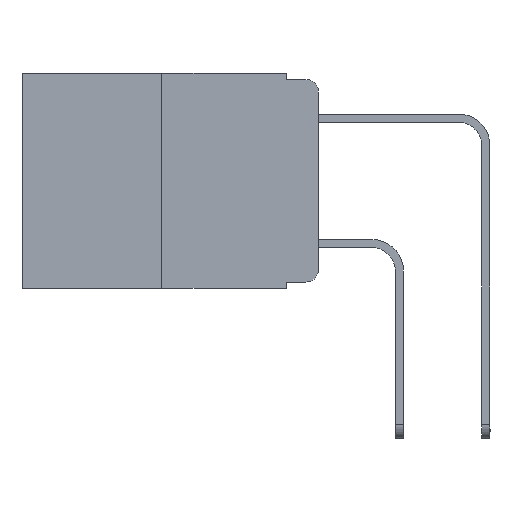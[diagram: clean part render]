
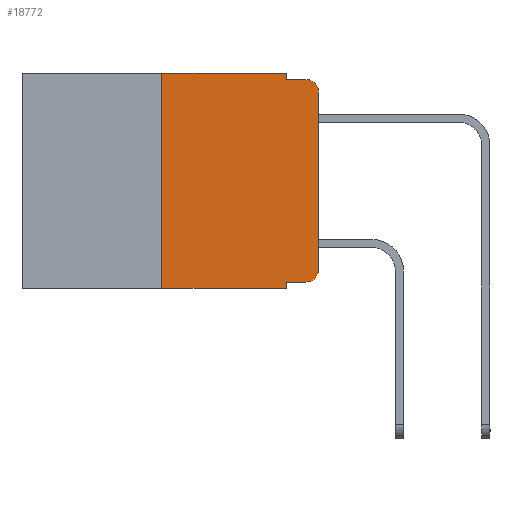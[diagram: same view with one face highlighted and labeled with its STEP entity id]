
A CAD part, left-side view. The second image highlights one B-rep face of the part: STEP entity #18772.
In plain terms, the highlighted planar face has unit normal (-1, 0, 0).
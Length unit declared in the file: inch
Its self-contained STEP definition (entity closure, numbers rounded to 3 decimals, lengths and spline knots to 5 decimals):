
#308 = DIRECTION ( 'NONE',  ( 0., 0., 1. ) ) ;
#322 = CARTESIAN_POINT ( 'NONE',  ( 0., 0.02, -0.333 ) ) ;
#410 = CARTESIAN_POINT ( 'NONE',  ( 0., 0.02, -0.313 ) ) ;
#515 = VECTOR ( 'NONE', #24752, 39.37008 ) ;
#552 = ORIENTED_EDGE ( 'NONE', *, *, #26550, .F. ) ;
#1046 = ORIENTED_EDGE ( 'NONE', *, *, #3903, .F. ) ;
#1959 = LINE ( 'NONE', #11991, #515 ) ;
#2117 = CARTESIAN_POINT ( 'NONE',  ( 0., 0.473, -0.343 ) ) ;
#2795 = VECTOR ( 'NONE', #3805, 39.37008 ) ;
#3055 = CARTESIAN_POINT ( 'NONE',  ( 0., 0.473, 0. ) ) ;
#3255 = CARTESIAN_POINT ( 'NONE',  ( 0., 0.051, -0.333 ) ) ;
#3805 = DIRECTION ( 'NONE',  ( 0., 0., -1. ) ) ;
#3903 = EDGE_CURVE ( 'NONE', #21490, #16347, #20404, .T. ) ;
#4224 = ORIENTED_EDGE ( 'NONE', *, *, #7014, .T. ) ;
#4335 = CARTESIAN_POINT ( 'NONE',  ( 0., 0., 0. ) ) ;
#4472 = LINE ( 'NONE', #4335, #6019 ) ;
#4534 = LINE ( 'NONE', #2117, #24745 ) ;
#4880 = AXIS2_PLACEMENT_3D ( 'NONE', #410, #16903, #4992 ) ;
#4992 = DIRECTION ( 'NONE',  ( 0., 0., -1. ) ) ;
#5060 = FACE_OUTER_BOUND ( 'NONE', #17353, .T. ) ;
#5159 = ORIENTED_EDGE ( 'NONE', *, *, #9480, .T. ) ;
#5389 = CARTESIAN_POINT ( 'NONE',  ( 0., 0.051, 0. ) ) ;
#5534 = DIRECTION ( 'NONE',  ( 0., 0., 1. ) ) ;
#6019 = VECTOR ( 'NONE', #308, 39.37008 ) ;
#6514 = ORIENTED_EDGE ( 'NONE', *, *, #7941, .F. ) ;
#7014 = EDGE_CURVE ( 'NONE', #9613, #23124, #14364, .T. ) ;
#7028 = VERTEX_POINT ( 'NONE', #19539 ) ;
#7389 = CARTESIAN_POINT ( 'NONE',  ( 0., 0.25, 0. ) ) ;
#7739 = ORIENTED_EDGE ( 'NONE', *, *, #18640, .T. ) ;
#7941 = EDGE_CURVE ( 'NONE', #16510, #10503, #19343, .T. ) ;
#8478 = VERTEX_POINT ( 'NONE', #9923 ) ;
#8979 = EDGE_CURVE ( 'NONE', #8478, #23124, #1959, .T. ) ;
#9098 = CARTESIAN_POINT ( 'NONE',  ( 0., 0.02, -0.01 ) ) ;
#9327 = DIRECTION ( 'NONE',  ( 1., 0., 0. ) ) ;
#9480 = EDGE_CURVE ( 'NONE', #16824, #7028, #12989, .T. ) ;
#9613 = VERTEX_POINT ( 'NONE', #15568 ) ;
#9795 = LINE ( 'NONE', #14210, #12015 ) ;
#9923 = CARTESIAN_POINT ( 'NONE',  ( 0., 0.051, -0.01 ) ) ;
#10267 = DIRECTION ( 'NONE',  ( 0., -1., 0. ) ) ;
#10503 = VERTEX_POINT ( 'NONE', #20475 ) ;
#11470 = PLANE ( 'NONE',  #24806 ) ;
#11743 = VECTOR ( 'NONE', #5534, 39.37008 ) ;
#11991 = CARTESIAN_POINT ( 'NONE',  ( 0., 0.051, -0.01 ) ) ;
#12015 = VECTOR ( 'NONE', #17972, 39.37008 ) ;
#12232 = CARTESIAN_POINT ( 'NONE',  ( 0., 0.051, 0. ) ) ;
#12686 = CARTESIAN_POINT ( 'NONE',  ( 0., 0.051, -0.343 ) ) ;
#12989 = CIRCLE ( 'NONE', #4880, 0.02 ) ;
#13209 = CARTESIAN_POINT ( 'NONE',  ( 0., 0.25, -0.343 ) ) ;
#13210 = ORIENTED_EDGE ( 'NONE', *, *, #8979, .F. ) ;
#14210 = CARTESIAN_POINT ( 'NONE',  ( 0., 0.051, 0. ) ) ;
#14364 = CIRCLE ( 'NONE', #23330, 0.02 ) ;
#15510 = DIRECTION ( 'NONE',  ( -1., 0., 0. ) ) ;
#15555 = DIRECTION ( 'NONE',  ( 0., -1., 0. ) ) ;
#15568 = CARTESIAN_POINT ( 'NONE',  ( 0., 0., -0.03 ) ) ;
#16347 = VERTEX_POINT ( 'NONE', #12686 ) ;
#16510 = VERTEX_POINT ( 'NONE', #13209 ) ;
#16783 = CARTESIAN_POINT ( 'NONE',  ( 0., 0.473, 0. ) ) ;
#16824 = VERTEX_POINT ( 'NONE', #322 ) ;
#16853 = ORIENTED_EDGE ( 'NONE', *, *, #21979, .T. ) ;
#16903 = DIRECTION ( 'NONE',  ( -1., 0., 0. ) ) ;
#16919 = LINE ( 'NONE', #16783, #18883 ) ;
#17353 = EDGE_LOOP ( 'NONE', ( #16853, #4224, #13210, #552, #26193, #6514, #7739, #1046, #21840, #5159 ) ) ;
#17803 = CARTESIAN_POINT ( 'NONE',  ( 0., 0.02, -0.03 ) ) ;
#17972 = DIRECTION ( 'NONE',  ( 0., 0., -1. ) ) ;
#18640 = EDGE_CURVE ( 'NONE', #16510, #16347, #4534, .T. ) ;
#18772 = ADVANCED_FACE ( 'NONE', ( #5060 ), #11470, .F. ) ;
#18883 = VECTOR ( 'NONE', #24995, 39.37008 ) ;
#19343 = LINE ( 'NONE', #7389, #11743 ) ;
#19385 = DIRECTION ( 'NONE',  ( 0., 0., -1. ) ) ;
#19539 = CARTESIAN_POINT ( 'NONE',  ( 0., 0., -0.313 ) ) ;
#20404 = LINE ( 'NONE', #12232, #2795 ) ;
#20475 = CARTESIAN_POINT ( 'NONE',  ( 0., 0.25, 0. ) ) ;
#21490 = VERTEX_POINT ( 'NONE', #26275 ) ;
#21819 = DIRECTION ( 'NONE',  ( 0., 0., -1. ) ) ;
#21840 = ORIENTED_EDGE ( 'NONE', *, *, #25826, .T. ) ;
#21979 = EDGE_CURVE ( 'NONE', #7028, #9613, #4472, .T. ) ;
#22005 = LINE ( 'NONE', #3255, #24438 ) ;
#23124 = VERTEX_POINT ( 'NONE', #9098 ) ;
#23330 = AXIS2_PLACEMENT_3D ( 'NONE', #17803, #15510, #21819 ) ;
#24438 = VECTOR ( 'NONE', #15555, 39.37008 ) ;
#24524 = VERTEX_POINT ( 'NONE', #5389 ) ;
#24745 = VECTOR ( 'NONE', #10267, 39.37008 ) ;
#24752 = DIRECTION ( 'NONE',  ( 0., -1., 0. ) ) ;
#24806 = AXIS2_PLACEMENT_3D ( 'NONE', #3055, #9327, #19385 ) ;
#24995 = DIRECTION ( 'NONE',  ( 0., -1., 0. ) ) ;
#25616 = EDGE_CURVE ( 'NONE', #10503, #24524, #16919, .T. ) ;
#25826 = EDGE_CURVE ( 'NONE', #21490, #16824, #22005, .T. ) ;
#26193 = ORIENTED_EDGE ( 'NONE', *, *, #25616, .F. ) ;
#26275 = CARTESIAN_POINT ( 'NONE',  ( 0., 0.051, -0.333 ) ) ;
#26550 = EDGE_CURVE ( 'NONE', #24524, #8478, #9795, .T. ) ;
